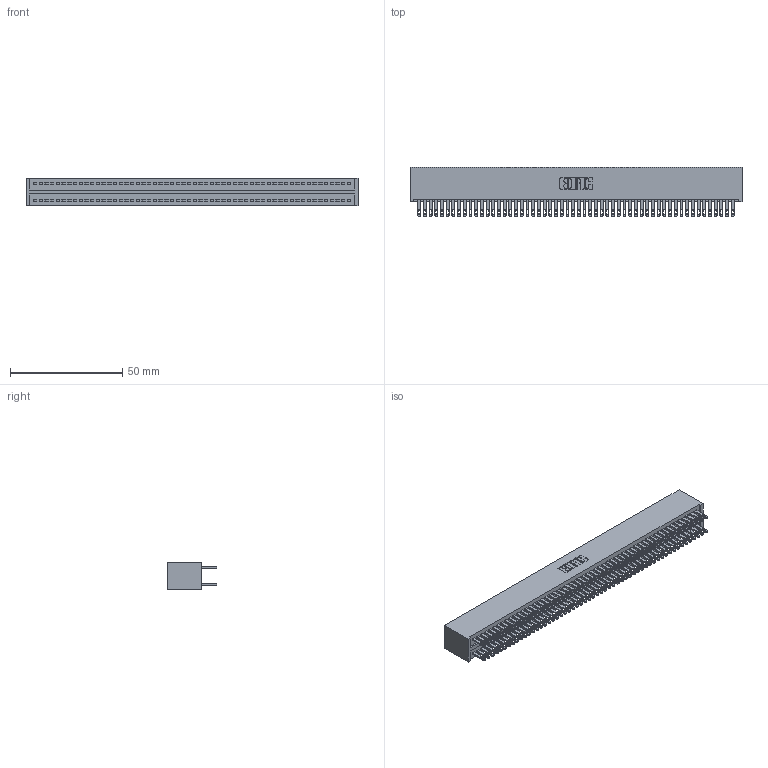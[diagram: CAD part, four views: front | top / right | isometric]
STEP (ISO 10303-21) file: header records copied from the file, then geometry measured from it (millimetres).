
FILE_DESCRIPTION (( 'STEP AP203' ), '1' );
FILE_NAME ('325-112-500-201.STEP', '2020-02-25T07:46:40', ( '' ), ( '' ), 'SwSTEP 2.0', 'SolidWorks 2016', '' );
FILE_SCHEMA (( 'CONFIG_CONTROL_DESIGN' ));
Length unit declared in the file: inch
Products named in the file (3): 325-292-001_325-293-100; 325 Part_Lugless; 325-112-500-201
Assembly tree (113 placements, depth 2):
  325-112-500-201
    325 Part_Lugless
    325-292-001_325-293-100  x112
Bounding box: 147.88 x 21.84 x 12.45 mm (x, y, z)
Volume: 20164.6 mm3; surface area: 26570.6 mm2
Topology: 113 solids, 113 shells, 5482 faces, 16751 edges, 11166 vertices
Faces by surface type: plane 3426, cylinder 2056
Entity records: 33869 total; most frequent: CARTESIAN_POINT 5594, ORIENTED_EDGE 5530, DIRECTION 4749, EDGE_CURVE 2765, LINE 2641, VECTOR 2641, VERTEX_POINT 1842, AXIS2_PLACEMENT_3D 1054
